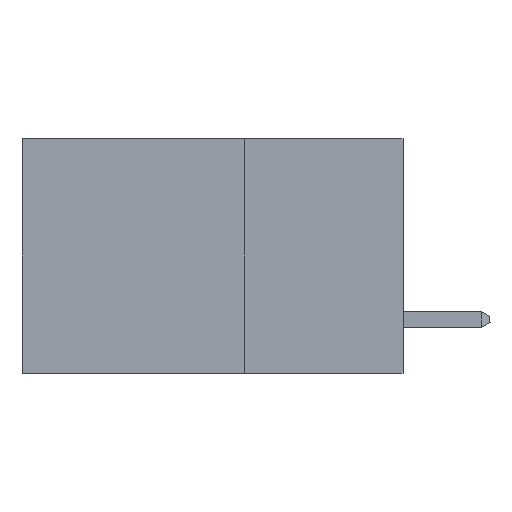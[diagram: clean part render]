
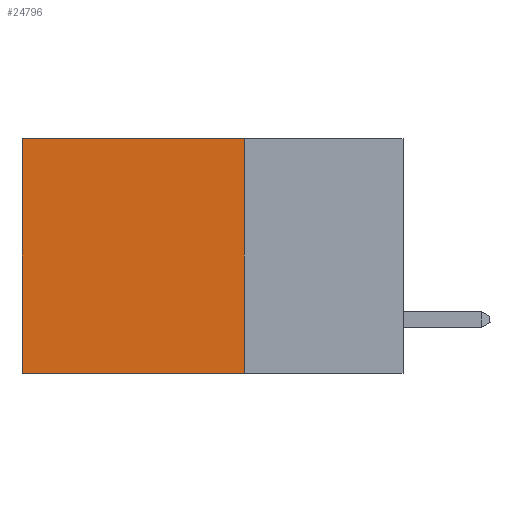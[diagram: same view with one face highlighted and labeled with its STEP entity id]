
A CAD part, left-side view. The second image highlights one B-rep face of the part: STEP entity #24796.
In plain terms, the highlighted planar face has unit normal (-1, 0, 0).
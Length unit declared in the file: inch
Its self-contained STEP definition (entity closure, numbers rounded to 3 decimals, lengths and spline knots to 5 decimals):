
#327 = ORIENTED_EDGE ( 'NONE', *, *, #40048, .T. ) ;
#404 = CARTESIAN_POINT ( 'NONE',  ( 0.2875, 0.25, -0.37 ) ) ;
#1080 = CARTESIAN_POINT ( 'NONE',  ( 0.2875, 0.25, 0. ) ) ;
#1096 = VERTEX_POINT ( 'NONE', #12206 ) ;
#3127 = CARTESIAN_POINT ( 'NONE',  ( 0.2875, 0.25, 0. ) ) ;
#3773 = EDGE_CURVE ( 'NONE', #38040, #37865, #7230, .T. ) ;
#3962 = VERTEX_POINT ( 'NONE', #404 ) ;
#4014 = EDGE_LOOP ( 'NONE', ( #30488, #23682, #31893, #327 ) ) ;
#4332 = DIRECTION ( 'NONE',  ( 0., 0., -1. ) ) ;
#4800 = LINE ( 'NONE', #30961, #29527 ) ;
#5510 = LINE ( 'NONE', #1080, #31225 ) ;
#6343 = DIRECTION ( 'NONE',  ( 0., 0., -1. ) ) ;
#6477 = EDGE_CURVE ( 'NONE', #1096, #3962, #5510, .T. ) ;
#7230 = LINE ( 'NONE', #16409, #39327 ) ;
#11814 = FACE_OUTER_BOUND ( 'NONE', #4014, .T. ) ;
#12206 = CARTESIAN_POINT ( 'NONE',  ( 0.2875, 0.25, 0. ) ) ;
#13504 = LINE ( 'NONE', #36062, #29723 ) ;
#16409 = CARTESIAN_POINT ( 'NONE',  ( 0.2875, 0.6, 0. ) ) ;
#18755 = AXIS2_PLACEMENT_3D ( 'NONE', #3127, #25666, #6343 ) ;
#21408 = DIRECTION ( 'NONE',  ( 0., 1., 0. ) ) ;
#23682 = ORIENTED_EDGE ( 'NONE', *, *, #29404, .F. ) ;
#24796 = ADVANCED_FACE ( 'NONE', ( #11814 ), #31982, .F. ) ;
#25666 = DIRECTION ( 'NONE',  ( 1., 0., 0. ) ) ;
#29404 = EDGE_CURVE ( 'NONE', #3962, #37865, #4800, .T. ) ;
#29527 = VECTOR ( 'NONE', #21408, 39.37008 ) ;
#29723 = VECTOR ( 'NONE', #39232, 39.37008 ) ;
#30488 = ORIENTED_EDGE ( 'NONE', *, *, #3773, .T. ) ;
#30961 = CARTESIAN_POINT ( 'NONE',  ( 0.2875, 0.25, -0.37 ) ) ;
#31225 = VECTOR ( 'NONE', #4332, 39.37008 ) ;
#31893 = ORIENTED_EDGE ( 'NONE', *, *, #6477, .F. ) ;
#31982 = PLANE ( 'NONE',  #18755 ) ;
#32445 = DIRECTION ( 'NONE',  ( 0., 0., -1. ) ) ;
#32876 = CARTESIAN_POINT ( 'NONE',  ( 0.2875, 0.6, 0. ) ) ;
#36062 = CARTESIAN_POINT ( 'NONE',  ( 0.2875, 0.25, 0. ) ) ;
#37865 = VERTEX_POINT ( 'NONE', #38274 ) ;
#38040 = VERTEX_POINT ( 'NONE', #32876 ) ;
#38274 = CARTESIAN_POINT ( 'NONE',  ( 0.2875, 0.6, -0.37 ) ) ;
#39232 = DIRECTION ( 'NONE',  ( 0., 1., 0. ) ) ;
#39327 = VECTOR ( 'NONE', #32445, 39.37008 ) ;
#40048 = EDGE_CURVE ( 'NONE', #1096, #38040, #13504, .T. ) ;
